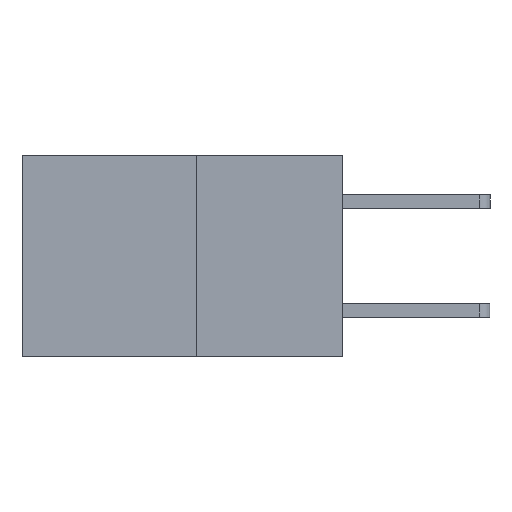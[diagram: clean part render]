
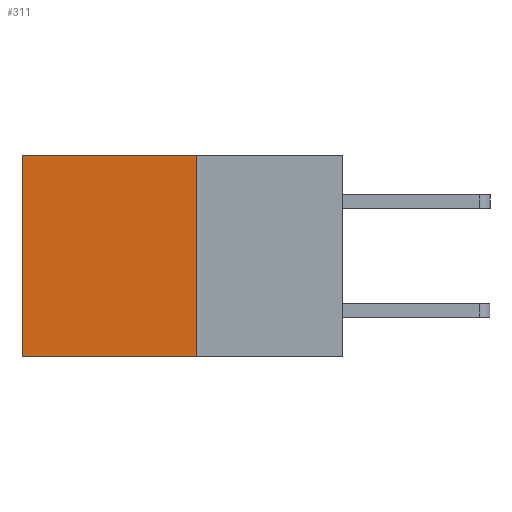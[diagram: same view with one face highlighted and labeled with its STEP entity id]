
A CAD part, left-side view. The second image highlights one B-rep face of the part: STEP entity #311.
In plain terms, the highlighted planar face has unit normal (-1, 0, 0).
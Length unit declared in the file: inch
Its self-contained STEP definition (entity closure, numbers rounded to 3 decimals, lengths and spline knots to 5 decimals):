
#108 = EDGE_CURVE ( 'NONE', #6718, #7824, #3503, .T. ) ;
#114 = DIRECTION ( 'NONE',  ( 0., 1., 0. ) ) ;
#311 = ADVANCED_FACE ( 'NONE', ( #4080 ), #2544, .F. ) ;
#350 = ORIENTED_EDGE ( 'NONE', *, *, #4856, .T. ) ;
#556 = VECTOR ( 'NONE', #4516, 39.37008 ) ;
#655 = VECTOR ( 'NONE', #6093, 39.37008 ) ;
#666 = ORIENTED_EDGE ( 'NONE', *, *, #5734, .F. ) ;
#1336 = CARTESIAN_POINT ( 'NONE',  ( 0.277, 0.27, -0.37 ) ) ;
#1457 = LINE ( 'NONE', #2135, #4565 ) ;
#1469 = CARTESIAN_POINT ( 'NONE',  ( 0.277, 0.59, -0.37 ) ) ;
#1559 = VERTEX_POINT ( 'NONE', #5231 ) ;
#1972 = ORIENTED_EDGE ( 'NONE', *, *, #2546, .T. ) ;
#2131 = ORIENTED_EDGE ( 'NONE', *, *, #108, .F. ) ;
#2135 = CARTESIAN_POINT ( 'NONE',  ( 0.277, 0.27, -0.37 ) ) ;
#2314 = VERTEX_POINT ( 'NONE', #1469 ) ;
#2544 = PLANE ( 'NONE',  #5200 ) ;
#2546 = EDGE_CURVE ( 'NONE', #6718, #1559, #3457, .T. ) ;
#3092 = CARTESIAN_POINT ( 'NONE',  ( 0.277, 0.27, -0.37 ) ) ;
#3457 = LINE ( 'NONE', #6738, #655 ) ;
#3503 = LINE ( 'NONE', #3092, #7552 ) ;
#3618 = DIRECTION ( 'NONE',  ( 0., 0., -1. ) ) ;
#4080 = FACE_OUTER_BOUND ( 'NONE', #4353, .T. ) ;
#4353 = EDGE_LOOP ( 'NONE', ( #350, #666, #2131, #1972 ) ) ;
#4516 = DIRECTION ( 'NONE',  ( 0., 0., -1. ) ) ;
#4565 = VECTOR ( 'NONE', #114, 39.37008 ) ;
#4856 = EDGE_CURVE ( 'NONE', #1559, #2314, #6939, .T. ) ;
#5200 = AXIS2_PLACEMENT_3D ( 'NONE', #5443, #5442, #3618 ) ;
#5231 = CARTESIAN_POINT ( 'NONE',  ( 0.277, 0.59, 0. ) ) ;
#5372 = DIRECTION ( 'NONE',  ( 0., 0., -1. ) ) ;
#5442 = DIRECTION ( 'NONE',  ( 1., 0., 0. ) ) ;
#5443 = CARTESIAN_POINT ( 'NONE',  ( 0.277, 0.27, -0.37 ) ) ;
#5726 = CARTESIAN_POINT ( 'NONE',  ( 0.277, 0.59, -0.37 ) ) ;
#5734 = EDGE_CURVE ( 'NONE', #7824, #2314, #1457, .T. ) ;
#6093 = DIRECTION ( 'NONE',  ( 0., 1., 0. ) ) ;
#6341 = CARTESIAN_POINT ( 'NONE',  ( 0.277, 0.27, 0. ) ) ;
#6718 = VERTEX_POINT ( 'NONE', #6341 ) ;
#6738 = CARTESIAN_POINT ( 'NONE',  ( 0.277, 0.27, 0. ) ) ;
#6939 = LINE ( 'NONE', #5726, #556 ) ;
#7552 = VECTOR ( 'NONE', #5372, 39.37008 ) ;
#7824 = VERTEX_POINT ( 'NONE', #1336 ) ;
